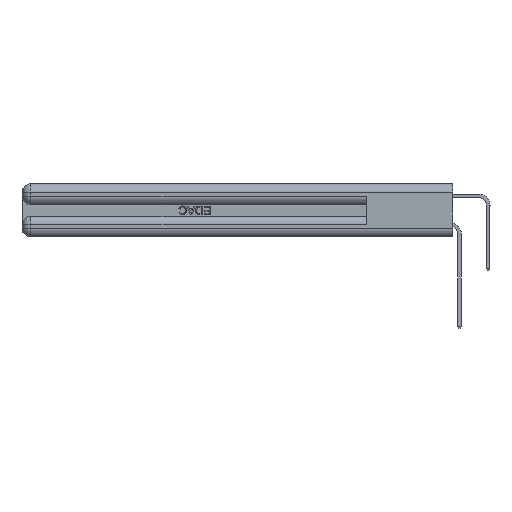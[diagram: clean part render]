
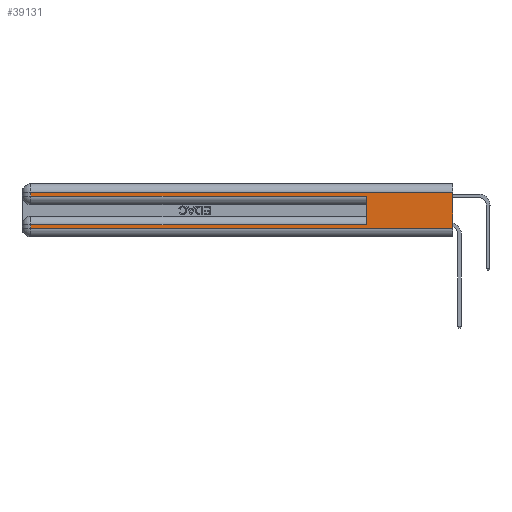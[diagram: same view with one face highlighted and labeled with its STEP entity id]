
A CAD part, left-side view. The second image highlights one B-rep face of the part: STEP entity #39131.
In plain terms, the highlighted planar face has unit normal (-1, 0, 0).
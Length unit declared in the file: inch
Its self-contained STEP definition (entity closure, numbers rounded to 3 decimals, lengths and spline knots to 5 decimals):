
#227 = CARTESIAN_POINT ( 'NONE',  ( 0., 2.94, 0.085 ) ) ;
#877 = VECTOR ( 'NONE', #49300, 39.37008 ) ;
#1200 = VECTOR ( 'NONE', #35318, 39.37008 ) ;
#1537 = VERTEX_POINT ( 'NONE', #31546 ) ;
#1715 = CARTESIAN_POINT ( 'NONE',  ( 0., 2.94, 0.37 ) ) ;
#4897 = CARTESIAN_POINT ( 'NONE',  ( 0., 0.6, 0.085 ) ) ;
#5176 = ORIENTED_EDGE ( 'NONE', *, *, #19854, .T. ) ;
#6411 = DIRECTION ( 'NONE',  ( 0., 1., 0. ) ) ;
#6791 = CARTESIAN_POINT ( 'NONE',  ( 0., 0., 0.085 ) ) ;
#6825 = CARTESIAN_POINT ( 'NONE',  ( 0., 0.6, 0.285 ) ) ;
#8571 = EDGE_CURVE ( 'NONE', #43367, #47031, #42185, .T. ) ;
#9190 = EDGE_CURVE ( 'NONE', #27422, #42495, #42707, .T. ) ;
#10988 = VECTOR ( 'NONE', #37869, 39.37008 ) ;
#11455 = FACE_OUTER_BOUND ( 'NONE', #44624, .T. ) ;
#12067 = CARTESIAN_POINT ( 'NONE',  ( 0., 0.6, 0.145 ) ) ;
#12147 = ORIENTED_EDGE ( 'NONE', *, *, #27176, .T. ) ;
#12235 = LINE ( 'NONE', #1715, #48567 ) ;
#13313 = VERTEX_POINT ( 'NONE', #27735 ) ;
#13633 = DIRECTION ( 'NONE',  ( 0., 0., -1. ) ) ;
#15478 = EDGE_CURVE ( 'NONE', #13313, #26652, #16910, .T. ) ;
#16699 = DIRECTION ( 'NONE',  ( 0., 0., -1. ) ) ;
#16910 = LINE ( 'NONE', #36045, #46595 ) ;
#19854 = EDGE_CURVE ( 'NONE', #1537, #27422, #41906, .T. ) ;
#19943 = VERTEX_POINT ( 'NONE', #41880 ) ;
#20089 = EDGE_CURVE ( 'NONE', #43367, #42495, #31001, .T. ) ;
#20877 = ORIENTED_EDGE ( 'NONE', *, *, #28141, .T. ) ;
#21228 = PLANE ( 'NONE',  #27870 ) ;
#22556 = CARTESIAN_POINT ( 'NONE',  ( 0., 0., 0.285 ) ) ;
#22622 = VECTOR ( 'NONE', #40114, 39.37008 ) ;
#22715 = DIRECTION ( 'NONE',  ( 0., -1., 0. ) ) ;
#23036 = ORIENTED_EDGE ( 'NONE', *, *, #15478, .F. ) ;
#24513 = ORIENTED_EDGE ( 'NONE', *, *, #20089, .F. ) ;
#24958 = CARTESIAN_POINT ( 'NONE',  ( 0., 0., 0.37 ) ) ;
#25080 = LINE ( 'NONE', #33564, #34175 ) ;
#25123 = DIRECTION ( 'NONE',  ( 0., 0., -1. ) ) ;
#26652 = VERTEX_POINT ( 'NONE', #33774 ) ;
#27176 = EDGE_CURVE ( 'NONE', #13313, #1537, #25080, .T. ) ;
#27422 = VERTEX_POINT ( 'NONE', #38984 ) ;
#27648 = EDGE_CURVE ( 'NONE', #19943, #26652, #44390, .T. ) ;
#27735 = CARTESIAN_POINT ( 'NONE',  ( 0., 0., 0.31 ) ) ;
#27870 = AXIS2_PLACEMENT_3D ( 'NONE', #24958, #48277, #25123 ) ;
#28141 = EDGE_CURVE ( 'NONE', #47031, #19943, #12235, .T. ) ;
#30238 = ORIENTED_EDGE ( 'NONE', *, *, #9190, .T. ) ;
#31001 = LINE ( 'NONE', #12067, #1200 ) ;
#31546 = CARTESIAN_POINT ( 'NONE',  ( 0., 2.94, 0.31 ) ) ;
#32353 = ORIENTED_EDGE ( 'NONE', *, *, #27648, .T. ) ;
#32425 = VECTOR ( 'NONE', #22715, 39.37008 ) ;
#33564 = CARTESIAN_POINT ( 'NONE',  ( 0., 0., 0.31 ) ) ;
#33774 = CARTESIAN_POINT ( 'NONE',  ( 0., 0., 0.06 ) ) ;
#33956 = CARTESIAN_POINT ( 'NONE',  ( 0., 2.94, 0.37 ) ) ;
#34175 = VECTOR ( 'NONE', #6411, 39.37008 ) ;
#35318 = DIRECTION ( 'NONE',  ( 0., 0., 1. ) ) ;
#36045 = CARTESIAN_POINT ( 'NONE',  ( 0., 0., 0.37 ) ) ;
#37869 = DIRECTION ( 'NONE',  ( 0., 0., -1. ) ) ;
#38984 = CARTESIAN_POINT ( 'NONE',  ( 0., 2.94, 0.285 ) ) ;
#39131 = ADVANCED_FACE ( 'NONE', ( #11455 ), #21228, .F. ) ;
#40064 = ORIENTED_EDGE ( 'NONE', *, *, #8571, .T. ) ;
#40114 = DIRECTION ( 'NONE',  ( 0., -1., 0. ) ) ;
#41880 = CARTESIAN_POINT ( 'NONE',  ( 0., 2.94, 0.06 ) ) ;
#41906 = LINE ( 'NONE', #33956, #10988 ) ;
#42185 = LINE ( 'NONE', #6791, #877 ) ;
#42495 = VERTEX_POINT ( 'NONE', #6825 ) ;
#42707 = LINE ( 'NONE', #22556, #32425 ) ;
#43367 = VERTEX_POINT ( 'NONE', #4897 ) ;
#43996 = CARTESIAN_POINT ( 'NONE',  ( 0., 0., 0.06 ) ) ;
#44390 = LINE ( 'NONE', #43996, #22622 ) ;
#44624 = EDGE_LOOP ( 'NONE', ( #23036, #12147, #5176, #30238, #24513, #40064, #20877, #32353 ) ) ;
#46595 = VECTOR ( 'NONE', #16699, 39.37008 ) ;
#47031 = VERTEX_POINT ( 'NONE', #227 ) ;
#48277 = DIRECTION ( 'NONE',  ( 1., 0., 0. ) ) ;
#48567 = VECTOR ( 'NONE', #13633, 39.37008 ) ;
#49300 = DIRECTION ( 'NONE',  ( 0., 1., 0. ) ) ;
